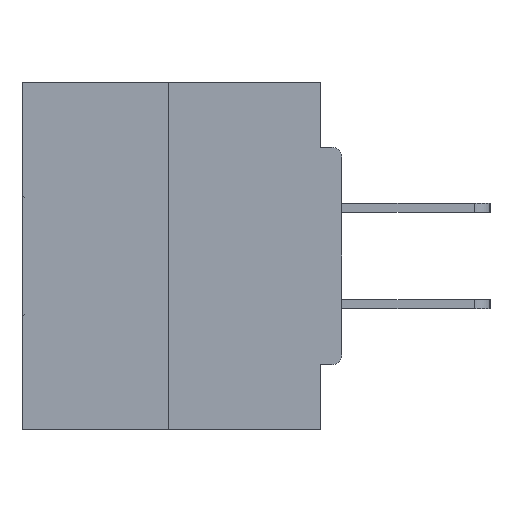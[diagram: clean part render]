
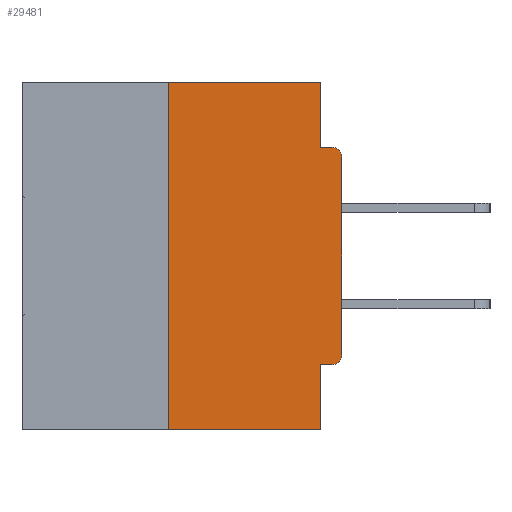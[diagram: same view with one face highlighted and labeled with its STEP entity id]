
A CAD part, left-side view. The second image highlights one B-rep face of the part: STEP entity #29481.
In plain terms, the highlighted planar face has unit normal (-1, 0, 0).
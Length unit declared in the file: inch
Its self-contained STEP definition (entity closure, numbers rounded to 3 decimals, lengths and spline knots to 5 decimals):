
#680 = CIRCLE ( 'NONE', #8310, 0.015 ) ;
#839 = DIRECTION ( 'NONE',  ( 0., 0., -1. ) ) ;
#1569 = CARTESIAN_POINT ( 'NONE',  ( 0., 0., -0.4065 ) ) ;
#1631 = CIRCLE ( 'NONE', #7680, 0.015 ) ;
#1849 = VERTEX_POINT ( 'NONE', #3960 ) ;
#2159 = VERTEX_POINT ( 'NONE', #29190 ) ;
#2928 = LINE ( 'NONE', #34426, #32131 ) ;
#3960 = CARTESIAN_POINT ( 'NONE',  ( 0., 0.031, -0.5 ) ) ;
#4293 = CARTESIAN_POINT ( 'NONE',  ( 0., 0.015, -0.0935 ) ) ;
#5369 = DIRECTION ( 'NONE',  ( 0., -1., 0. ) ) ;
#5887 = VECTOR ( 'NONE', #29958, 39.37008 ) ;
#7290 = ORIENTED_EDGE ( 'NONE', *, *, #27679, .F. ) ;
#7464 = EDGE_CURVE ( 'NONE', #2159, #40471, #38307, .T. ) ;
#7468 = CARTESIAN_POINT ( 'NONE',  ( 0., 0.015, -0.3915 ) ) ;
#7680 = AXIS2_PLACEMENT_3D ( 'NONE', #23085, #40239, #30392 ) ;
#8310 = AXIS2_PLACEMENT_3D ( 'NONE', #7468, #30101, #29954 ) ;
#8370 = CARTESIAN_POINT ( 'NONE',  ( 0., 0.46, -0.5 ) ) ;
#9057 = LINE ( 'NONE', #13665, #29160 ) ;
#9157 = ORIENTED_EDGE ( 'NONE', *, *, #18513, .F. ) ;
#11484 = VECTOR ( 'NONE', #24826, 39.37008 ) ;
#12638 = VECTOR ( 'NONE', #37041, 39.37008 ) ;
#13665 = CARTESIAN_POINT ( 'NONE',  ( 0., 0.031, -0.5 ) ) ;
#14090 = CARTESIAN_POINT ( 'NONE',  ( 0., 0., -0.3915 ) ) ;
#15087 = DIRECTION ( 'NONE',  ( 0., -1., 0. ) ) ;
#15545 = ORIENTED_EDGE ( 'NONE', *, *, #40912, .F. ) ;
#15553 = EDGE_CURVE ( 'NONE', #22252, #30674, #1631, .T. ) ;
#15722 = VECTOR ( 'NONE', #17397, 39.37008 ) ;
#16675 = ORIENTED_EDGE ( 'NONE', *, *, #19502, .F. ) ;
#16812 = PLANE ( 'NONE',  #32493 ) ;
#16959 = LINE ( 'NONE', #41102, #11484 ) ;
#17118 = CARTESIAN_POINT ( 'NONE',  ( 0., 0.46, 0. ) ) ;
#17397 = DIRECTION ( 'NONE',  ( 0., 0., -1. ) ) ;
#17432 = EDGE_CURVE ( 'NONE', #32766, #1849, #9057, .T. ) ;
#18394 = CARTESIAN_POINT ( 'NONE',  ( 0., 0.031, -0.4065 ) ) ;
#18513 = EDGE_CURVE ( 'NONE', #28762, #30674, #2928, .T. ) ;
#19030 = EDGE_CURVE ( 'NONE', #25563, #22252, #16959, .T. ) ;
#19502 = EDGE_CURVE ( 'NONE', #40471, #38047, #26066, .T. ) ;
#20834 = EDGE_CURVE ( 'NONE', #29019, #25563, #680, .T. ) ;
#22078 = CARTESIAN_POINT ( 'NONE',  ( 0., 0.031, 0. ) ) ;
#22252 = VERTEX_POINT ( 'NONE', #26545 ) ;
#23085 = CARTESIAN_POINT ( 'NONE',  ( 0., 0.015, -0.1085 ) ) ;
#24620 = VECTOR ( 'NONE', #5369, 39.37008 ) ;
#24826 = DIRECTION ( 'NONE',  ( 0., 0., 1. ) ) ;
#25060 = EDGE_CURVE ( 'NONE', #2159, #1849, #41693, .T. ) ;
#25563 = VERTEX_POINT ( 'NONE', #14090 ) ;
#26066 = LINE ( 'NONE', #17118, #5887 ) ;
#26488 = CARTESIAN_POINT ( 'NONE',  ( 0., 0.031, -0.0935 ) ) ;
#26545 = CARTESIAN_POINT ( 'NONE',  ( 0., 0., -0.1085 ) ) ;
#26718 = EDGE_LOOP ( 'NONE', ( #16675, #33657, #30423, #37826, #15545, #38203, #30394, #31781, #9157, #7290 ) ) ;
#27368 = CARTESIAN_POINT ( 'NONE',  ( 0., 0.25, 0. ) ) ;
#27679 = EDGE_CURVE ( 'NONE', #38047, #28762, #31405, .T. ) ;
#28762 = VERTEX_POINT ( 'NONE', #26488 ) ;
#29019 = VERTEX_POINT ( 'NONE', #34486 ) ;
#29160 = VECTOR ( 'NONE', #839, 39.37008 ) ;
#29190 = CARTESIAN_POINT ( 'NONE',  ( 0., 0.25, -0.5 ) ) ;
#29481 = ADVANCED_FACE ( 'NONE', ( #29726 ), #16812, .F. ) ;
#29726 = FACE_OUTER_BOUND ( 'NONE', #26718, .T. ) ;
#29954 = DIRECTION ( 'NONE',  ( 0., 0., -1. ) ) ;
#29958 = DIRECTION ( 'NONE',  ( 0., -1., 0. ) ) ;
#30086 = CARTESIAN_POINT ( 'NONE',  ( 0., 0.031, 0. ) ) ;
#30101 = DIRECTION ( 'NONE',  ( -1., 0., 0. ) ) ;
#30392 = DIRECTION ( 'NONE',  ( 0., 0., -1. ) ) ;
#30394 = ORIENTED_EDGE ( 'NONE', *, *, #19030, .T. ) ;
#30423 = ORIENTED_EDGE ( 'NONE', *, *, #25060, .T. ) ;
#30590 = DIRECTION ( 'NONE',  ( 0., 1., 0. ) ) ;
#30627 = CARTESIAN_POINT ( 'NONE',  ( 0., 0.25, 0. ) ) ;
#30674 = VERTEX_POINT ( 'NONE', #4293 ) ;
#31405 = LINE ( 'NONE', #30086, #15722 ) ;
#31781 = ORIENTED_EDGE ( 'NONE', *, *, #15553, .T. ) ;
#32131 = VECTOR ( 'NONE', #15087, 39.37008 ) ;
#32493 = AXIS2_PLACEMENT_3D ( 'NONE', #39352, #33037, #33319 ) ;
#32766 = VERTEX_POINT ( 'NONE', #18394 ) ;
#33037 = DIRECTION ( 'NONE',  ( 1., 0., 0. ) ) ;
#33319 = DIRECTION ( 'NONE',  ( 0., 0., -1. ) ) ;
#33657 = ORIENTED_EDGE ( 'NONE', *, *, #7464, .F. ) ;
#33842 = VECTOR ( 'NONE', #30590, 39.37008 ) ;
#34426 = CARTESIAN_POINT ( 'NONE',  ( 0., 0., -0.0935 ) ) ;
#34486 = CARTESIAN_POINT ( 'NONE',  ( 0., 0.015, -0.4065 ) ) ;
#37041 = DIRECTION ( 'NONE',  ( 0., 0., 1. ) ) ;
#37368 = LINE ( 'NONE', #1569, #33842 ) ;
#37826 = ORIENTED_EDGE ( 'NONE', *, *, #17432, .F. ) ;
#38047 = VERTEX_POINT ( 'NONE', #22078 ) ;
#38203 = ORIENTED_EDGE ( 'NONE', *, *, #20834, .T. ) ;
#38307 = LINE ( 'NONE', #27368, #12638 ) ;
#39352 = CARTESIAN_POINT ( 'NONE',  ( 0., 0.46, 0. ) ) ;
#40239 = DIRECTION ( 'NONE',  ( -1., 0., 0. ) ) ;
#40471 = VERTEX_POINT ( 'NONE', #30627 ) ;
#40912 = EDGE_CURVE ( 'NONE', #29019, #32766, #37368, .T. ) ;
#41102 = CARTESIAN_POINT ( 'NONE',  ( 0., 0., 0. ) ) ;
#41693 = LINE ( 'NONE', #8370, #24620 ) ;
